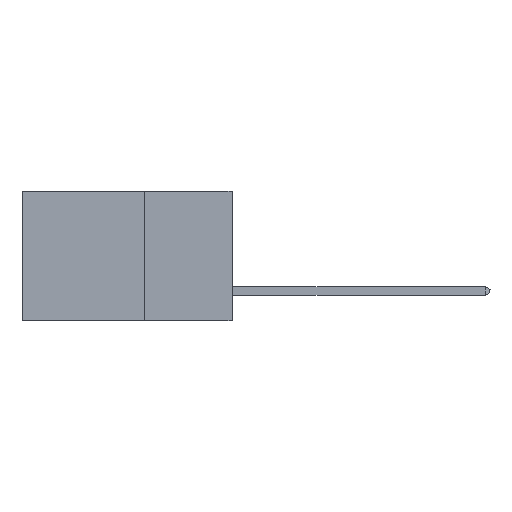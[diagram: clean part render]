
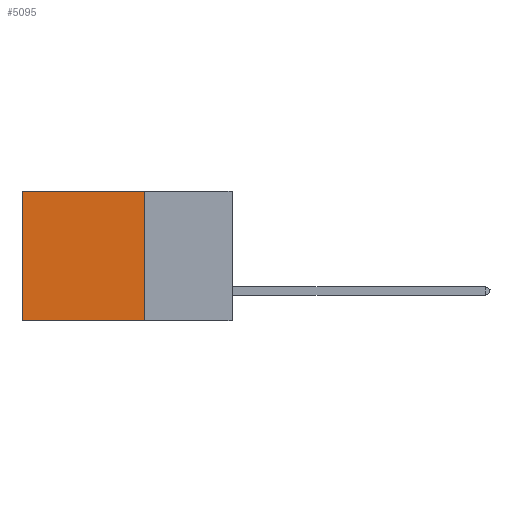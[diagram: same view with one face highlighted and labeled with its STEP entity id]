
A CAD part, left-side view. The second image highlights one B-rep face of the part: STEP entity #5095.
In plain terms, the highlighted planar face has unit normal (-1, 0, 0).
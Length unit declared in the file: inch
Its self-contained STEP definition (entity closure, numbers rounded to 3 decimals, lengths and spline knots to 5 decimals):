
#745 = CARTESIAN_POINT ( 'NONE',  ( 0.2875, 0.25, -0.37 ) ) ;
#1836 = VECTOR ( 'NONE', #33329, 39.37008 ) ;
#3578 = CARTESIAN_POINT ( 'NONE',  ( 0.2875, 0.25, -0.37 ) ) ;
#4947 = CARTESIAN_POINT ( 'NONE',  ( 0.2875, 0.25, 0. ) ) ;
#5095 = ADVANCED_FACE ( 'NONE', ( #24916 ), #35061, .F. ) ;
#5684 = VECTOR ( 'NONE', #27260, 39.37008 ) ;
#6564 = VERTEX_POINT ( 'NONE', #17032 ) ;
#7008 = VERTEX_POINT ( 'NONE', #33594 ) ;
#9049 = ORIENTED_EDGE ( 'NONE', *, *, #24037, .F. ) ;
#9191 = AXIS2_PLACEMENT_3D ( 'NONE', #9787, #29142, #34797 ) ;
#9787 = CARTESIAN_POINT ( 'NONE',  ( 0.2875, 0.25, 0. ) ) ;
#11911 = CARTESIAN_POINT ( 'NONE',  ( 0.2875, 0.25, 0. ) ) ;
#12423 = DIRECTION ( 'NONE',  ( 0., 0., -1. ) ) ;
#14415 = LINE ( 'NONE', #11911, #27814 ) ;
#14889 = VECTOR ( 'NONE', #23072, 39.37008 ) ;
#17032 = CARTESIAN_POINT ( 'NONE',  ( 0.2875, 0.6, 0. ) ) ;
#17939 = VERTEX_POINT ( 'NONE', #29695 ) ;
#17988 = EDGE_CURVE ( 'NONE', #6564, #17939, #22600, .T. ) ;
#19596 = EDGE_LOOP ( 'NONE', ( #29422, #9049, #33514, #20748 ) ) ;
#20748 = ORIENTED_EDGE ( 'NONE', *, *, #24276, .T. ) ;
#22600 = LINE ( 'NONE', #30382, #1836 ) ;
#23018 = LINE ( 'NONE', #3578, #14889 ) ;
#23072 = DIRECTION ( 'NONE',  ( 0., 1., 0. ) ) ;
#24037 = EDGE_CURVE ( 'NONE', #31310, #17939, #23018, .T. ) ;
#24276 = EDGE_CURVE ( 'NONE', #7008, #6564, #30397, .T. ) ;
#24916 = FACE_OUTER_BOUND ( 'NONE', #19596, .T. ) ;
#27260 = DIRECTION ( 'NONE',  ( 0., 1., 0. ) ) ;
#27814 = VECTOR ( 'NONE', #12423, 39.37008 ) ;
#27976 = EDGE_CURVE ( 'NONE', #7008, #31310, #14415, .T. ) ;
#29142 = DIRECTION ( 'NONE',  ( 1., 0., 0. ) ) ;
#29422 = ORIENTED_EDGE ( 'NONE', *, *, #17988, .T. ) ;
#29695 = CARTESIAN_POINT ( 'NONE',  ( 0.2875, 0.6, -0.37 ) ) ;
#30382 = CARTESIAN_POINT ( 'NONE',  ( 0.2875, 0.6, 0. ) ) ;
#30397 = LINE ( 'NONE', #4947, #5684 ) ;
#31310 = VERTEX_POINT ( 'NONE', #745 ) ;
#33329 = DIRECTION ( 'NONE',  ( 0., 0., -1. ) ) ;
#33514 = ORIENTED_EDGE ( 'NONE', *, *, #27976, .F. ) ;
#33594 = CARTESIAN_POINT ( 'NONE',  ( 0.2875, 0.25, 0. ) ) ;
#34797 = DIRECTION ( 'NONE',  ( 0., 0., -1. ) ) ;
#35061 = PLANE ( 'NONE',  #9191 ) ;
